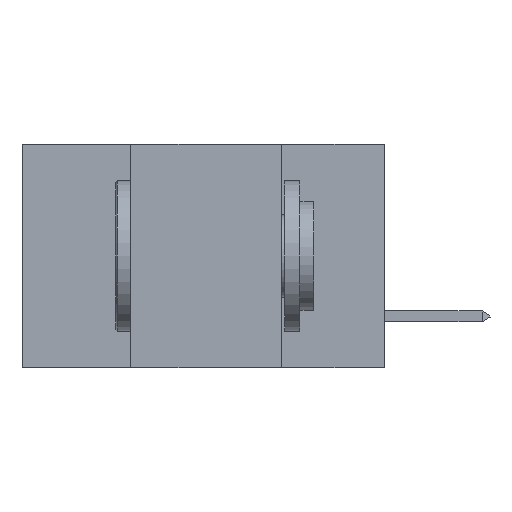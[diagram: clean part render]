
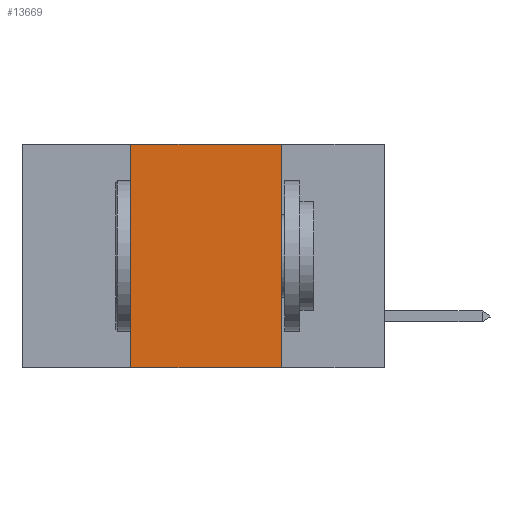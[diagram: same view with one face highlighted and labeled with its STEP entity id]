
A CAD part, left-side view. The second image highlights one B-rep face of the part: STEP entity #13669.
In plain terms, the highlighted planar face has unit normal (-1, 0, 0).
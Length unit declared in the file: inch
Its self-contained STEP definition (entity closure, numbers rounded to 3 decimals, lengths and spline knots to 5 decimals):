
#1541 = LINE ( 'NONE', #7716, #6332 ) ;
#1964 = DIRECTION ( 'NONE',  ( 0., 0., -1. ) ) ;
#3220 = CARTESIAN_POINT ( 'NONE',  ( 0., 0.6, 0. ) ) ;
#3366 = EDGE_CURVE ( 'NONE', #26070, #23014, #21477, .T. ) ;
#6332 = VECTOR ( 'NONE', #32933, 39.37008 ) ;
#7662 = VERTEX_POINT ( 'NONE', #31867 ) ;
#7716 = CARTESIAN_POINT ( 'NONE',  ( 0., 0.17, 0. ) ) ;
#10056 = ORIENTED_EDGE ( 'NONE', *, *, #23599, .F. ) ;
#10692 = CARTESIAN_POINT ( 'NONE',  ( 0., 0.17, -0.37 ) ) ;
#11239 = AXIS2_PLACEMENT_3D ( 'NONE', #15900, #32796, #1964 ) ;
#12601 = LINE ( 'NONE', #3220, #35790 ) ;
#12722 = VECTOR ( 'NONE', #25105, 39.37008 ) ;
#13669 = ADVANCED_FACE ( 'NONE', ( #14552 ), #32919, .F. ) ;
#13693 = VECTOR ( 'NONE', #17741, 39.37008 ) ;
#14202 = CARTESIAN_POINT ( 'NONE',  ( 0., 0.42, 0. ) ) ;
#14552 = FACE_OUTER_BOUND ( 'NONE', #14681, .T. ) ;
#14681 = EDGE_LOOP ( 'NONE', ( #10056, #32406, #19362, #24066 ) ) ;
#15900 = CARTESIAN_POINT ( 'NONE',  ( 0., 0.6, 0. ) ) ;
#16800 = EDGE_CURVE ( 'NONE', #26070, #31989, #24191, .T. ) ;
#17172 = DIRECTION ( 'NONE',  ( 0., -1., 0. ) ) ;
#17741 = DIRECTION ( 'NONE',  ( 0., 0., 1. ) ) ;
#19362 = ORIENTED_EDGE ( 'NONE', *, *, #16800, .F. ) ;
#21477 = LINE ( 'NONE', #33429, #12722 ) ;
#23014 = VERTEX_POINT ( 'NONE', #10692 ) ;
#23599 = EDGE_CURVE ( 'NONE', #7662, #23014, #1541, .T. ) ;
#24066 = ORIENTED_EDGE ( 'NONE', *, *, #3366, .T. ) ;
#24191 = LINE ( 'NONE', #14202, #13693 ) ;
#24604 = CARTESIAN_POINT ( 'NONE',  ( 0., 0.42, 0. ) ) ;
#25105 = DIRECTION ( 'NONE',  ( 0., -1., 0. ) ) ;
#26070 = VERTEX_POINT ( 'NONE', #30618 ) ;
#30618 = CARTESIAN_POINT ( 'NONE',  ( 0., 0.42, -0.37 ) ) ;
#31867 = CARTESIAN_POINT ( 'NONE',  ( 0., 0.17, 0. ) ) ;
#31989 = VERTEX_POINT ( 'NONE', #24604 ) ;
#32406 = ORIENTED_EDGE ( 'NONE', *, *, #32780, .F. ) ;
#32780 = EDGE_CURVE ( 'NONE', #31989, #7662, #12601, .T. ) ;
#32796 = DIRECTION ( 'NONE',  ( 1., 0., 0. ) ) ;
#32919 = PLANE ( 'NONE',  #11239 ) ;
#32933 = DIRECTION ( 'NONE',  ( 0., 0., -1. ) ) ;
#33429 = CARTESIAN_POINT ( 'NONE',  ( 0., 0.6, -0.37 ) ) ;
#35790 = VECTOR ( 'NONE', #17172, 39.37008 ) ;
